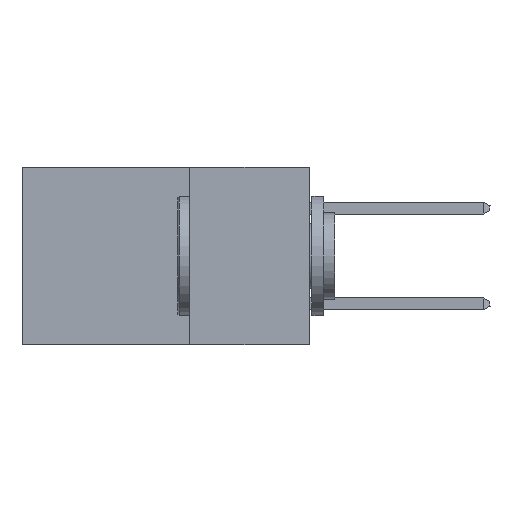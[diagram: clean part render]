
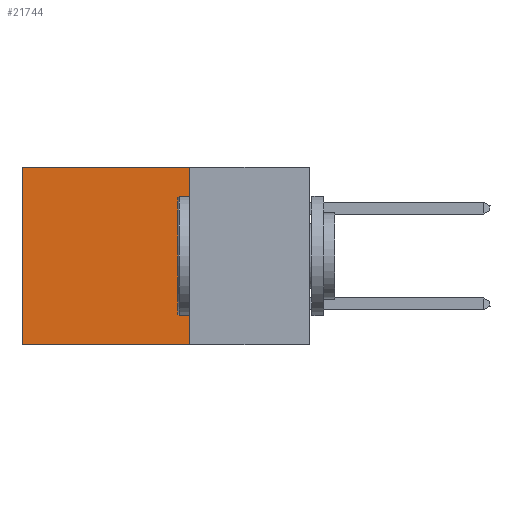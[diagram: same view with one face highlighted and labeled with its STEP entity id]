
A CAD part, left-side view. The second image highlights one B-rep face of the part: STEP entity #21744.
In plain terms, the highlighted planar face has unit normal (-1, 0, 0).
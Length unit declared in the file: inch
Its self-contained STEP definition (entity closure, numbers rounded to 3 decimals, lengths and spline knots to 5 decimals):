
#749 = EDGE_LOOP ( 'NONE', ( #13064, #8068, #10140, #21162 ) ) ;
#1655 = CARTESIAN_POINT ( 'NONE',  ( 0.2875, 0.25, -0.37 ) ) ;
#2583 = LINE ( 'NONE', #23029, #19734 ) ;
#3114 = DIRECTION ( 'NONE',  ( 0., 0., -1. ) ) ;
#3654 = AXIS2_PLACEMENT_3D ( 'NONE', #9898, #6290, #17999 ) ;
#6290 = DIRECTION ( 'NONE',  ( 1., 0., 0. ) ) ;
#7877 = DIRECTION ( 'NONE',  ( 0., 0., -1. ) ) ;
#8068 = ORIENTED_EDGE ( 'NONE', *, *, #13004, .F. ) ;
#8148 = LINE ( 'NONE', #20127, #8424 ) ;
#8424 = VECTOR ( 'NONE', #18546, 39.37008 ) ;
#8681 = LINE ( 'NONE', #12749, #19623 ) ;
#9215 = CARTESIAN_POINT ( 'NONE',  ( 0.2875, 0.6, 0. ) ) ;
#9898 = CARTESIAN_POINT ( 'NONE',  ( 0.2875, 0.25, 0. ) ) ;
#10140 = ORIENTED_EDGE ( 'NONE', *, *, #18758, .F. ) ;
#11195 = CARTESIAN_POINT ( 'NONE',  ( 0.2875, 0.25, 0. ) ) ;
#11769 = VECTOR ( 'NONE', #7877, 39.37008 ) ;
#12736 = FACE_OUTER_BOUND ( 'NONE', #749, .T. ) ;
#12749 = CARTESIAN_POINT ( 'NONE',  ( 0.2875, 0.25, -0.37 ) ) ;
#13004 = EDGE_CURVE ( 'NONE', #19568, #19265, #8681, .T. ) ;
#13064 = ORIENTED_EDGE ( 'NONE', *, *, #22655, .T. ) ;
#13742 = VERTEX_POINT ( 'NONE', #9215 ) ;
#13842 = PLANE ( 'NONE',  #3654 ) ;
#14729 = DIRECTION ( 'NONE',  ( 0., 1., 0. ) ) ;
#17999 = DIRECTION ( 'NONE',  ( 0., 0., -1. ) ) ;
#18296 = EDGE_CURVE ( 'NONE', #21827, #13742, #8148, .T. ) ;
#18546 = DIRECTION ( 'NONE',  ( 0., 1., 0. ) ) ;
#18758 = EDGE_CURVE ( 'NONE', #21827, #19568, #22418, .T. ) ;
#18839 = CARTESIAN_POINT ( 'NONE',  ( 0.2875, 0.25, 0. ) ) ;
#19265 = VERTEX_POINT ( 'NONE', #22268 ) ;
#19568 = VERTEX_POINT ( 'NONE', #1655 ) ;
#19623 = VECTOR ( 'NONE', #14729, 39.37008 ) ;
#19734 = VECTOR ( 'NONE', #3114, 39.37008 ) ;
#20127 = CARTESIAN_POINT ( 'NONE',  ( 0.2875, 0.25, 0. ) ) ;
#21162 = ORIENTED_EDGE ( 'NONE', *, *, #18296, .T. ) ;
#21744 = ADVANCED_FACE ( 'NONE', ( #12736 ), #13842, .F. ) ;
#21827 = VERTEX_POINT ( 'NONE', #18839 ) ;
#22268 = CARTESIAN_POINT ( 'NONE',  ( 0.2875, 0.6, -0.37 ) ) ;
#22418 = LINE ( 'NONE', #11195, #11769 ) ;
#22655 = EDGE_CURVE ( 'NONE', #13742, #19265, #2583, .T. ) ;
#23029 = CARTESIAN_POINT ( 'NONE',  ( 0.2875, 0.6, 0. ) ) ;
